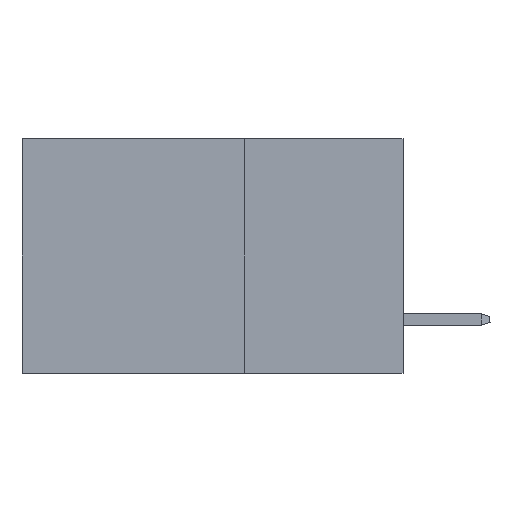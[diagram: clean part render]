
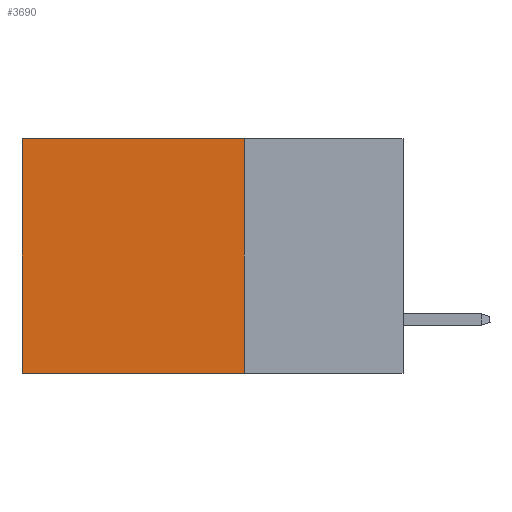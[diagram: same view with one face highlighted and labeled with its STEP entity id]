
A CAD part, left-side view. The second image highlights one B-rep face of the part: STEP entity #3690.
In plain terms, the highlighted planar face has unit normal (-1, 0, 0).
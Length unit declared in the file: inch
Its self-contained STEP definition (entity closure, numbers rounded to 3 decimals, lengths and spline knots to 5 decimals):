
#574 = VERTEX_POINT ( 'NONE', #26050 ) ;
#1919 = VERTEX_POINT ( 'NONE', #14316 ) ;
#2139 = VECTOR ( 'NONE', #34781, 39.37008 ) ;
#3690 = ADVANCED_FACE ( 'NONE', ( #39539 ), #4751, .F. ) ;
#3822 = VECTOR ( 'NONE', #25267, 39.37008 ) ;
#4751 = PLANE ( 'NONE',  #28431 ) ;
#5881 = EDGE_LOOP ( 'NONE', ( #15811, #40512, #35771, #25669 ) ) ;
#7143 = EDGE_CURVE ( 'NONE', #18458, #1919, #29170, .T. ) ;
#7786 = LINE ( 'NONE', #16910, #9262 ) ;
#8055 = DIRECTION ( 'NONE',  ( 1., 0., 0. ) ) ;
#9262 = VECTOR ( 'NONE', #19808, 39.37008 ) ;
#10283 = LINE ( 'NONE', #23339, #38850 ) ;
#13545 = EDGE_CURVE ( 'NONE', #18458, #36940, #37488, .T. ) ;
#14316 = CARTESIAN_POINT ( 'NONE',  ( 0.2875, 0.25, -0.37 ) ) ;
#15811 = ORIENTED_EDGE ( 'NONE', *, *, #31243, .T. ) ;
#16840 = CARTESIAN_POINT ( 'NONE',  ( 0.2875, 0.6, 0. ) ) ;
#16910 = CARTESIAN_POINT ( 'NONE',  ( 0.2875, 0.25, -0.37 ) ) ;
#18458 = VERTEX_POINT ( 'NONE', #26125 ) ;
#19638 = CARTESIAN_POINT ( 'NONE',  ( 0.2875, 0.25, 0. ) ) ;
#19808 = DIRECTION ( 'NONE',  ( 0., 1., 0. ) ) ;
#20679 = DIRECTION ( 'NONE',  ( 0., 0., -1. ) ) ;
#21738 = CARTESIAN_POINT ( 'NONE',  ( 0.2875, 0.25, 0. ) ) ;
#23339 = CARTESIAN_POINT ( 'NONE',  ( 0.2875, 0.6, 0. ) ) ;
#25267 = DIRECTION ( 'NONE',  ( 0., 1., 0. ) ) ;
#25669 = ORIENTED_EDGE ( 'NONE', *, *, #13545, .T. ) ;
#26050 = CARTESIAN_POINT ( 'NONE',  ( 0.2875, 0.6, -0.37 ) ) ;
#26125 = CARTESIAN_POINT ( 'NONE',  ( 0.2875, 0.25, 0. ) ) ;
#28431 = AXIS2_PLACEMENT_3D ( 'NONE', #36431, #8055, #20679 ) ;
#29170 = LINE ( 'NONE', #19638, #2139 ) ;
#31243 = EDGE_CURVE ( 'NONE', #36940, #574, #10283, .T. ) ;
#34781 = DIRECTION ( 'NONE',  ( 0., 0., -1. ) ) ;
#35771 = ORIENTED_EDGE ( 'NONE', *, *, #7143, .F. ) ;
#36431 = CARTESIAN_POINT ( 'NONE',  ( 0.2875, 0.25, 0. ) ) ;
#36940 = VERTEX_POINT ( 'NONE', #16840 ) ;
#37488 = LINE ( 'NONE', #21738, #3822 ) ;
#38569 = EDGE_CURVE ( 'NONE', #1919, #574, #7786, .T. ) ;
#38850 = VECTOR ( 'NONE', #38877, 39.37008 ) ;
#38877 = DIRECTION ( 'NONE',  ( 0., 0., -1. ) ) ;
#39539 = FACE_OUTER_BOUND ( 'NONE', #5881, .T. ) ;
#40512 = ORIENTED_EDGE ( 'NONE', *, *, #38569, .F. ) ;
